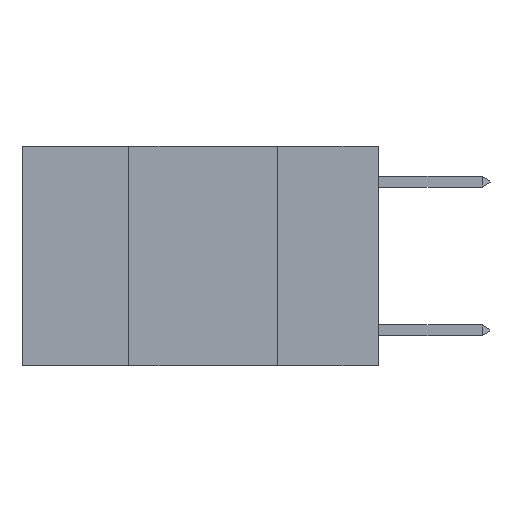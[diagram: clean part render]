
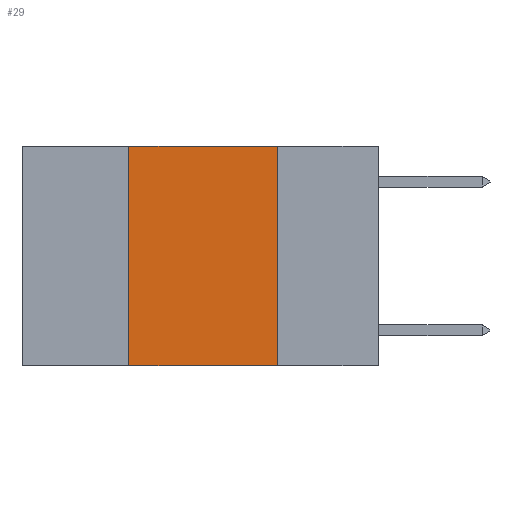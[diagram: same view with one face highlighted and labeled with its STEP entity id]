
A CAD part, left-side view. The second image highlights one B-rep face of the part: STEP entity #29.
In plain terms, the highlighted planar face has unit normal (-1, 0, 0).
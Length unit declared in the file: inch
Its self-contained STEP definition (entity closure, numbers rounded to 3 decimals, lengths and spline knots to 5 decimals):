
#29 = ADVANCED_FACE ( 'NONE', ( #16730 ), #16872, .F. ) ;
#124 = ORIENTED_EDGE ( 'NONE', *, *, #5923, .F. ) ;
#1288 = ORIENTED_EDGE ( 'NONE', *, *, #21244, .T. ) ;
#1526 = VERTEX_POINT ( 'NONE', #14755 ) ;
#2384 = ORIENTED_EDGE ( 'NONE', *, *, #12712, .F. ) ;
#3953 = LINE ( 'NONE', #10150, #18606 ) ;
#3977 = CARTESIAN_POINT ( 'NONE',  ( 0., 0.42, 0. ) ) ;
#5095 = VECTOR ( 'NONE', #12789, 39.37008 ) ;
#5812 = EDGE_LOOP ( 'NONE', ( #2384, #19786, #124, #1288 ) ) ;
#5857 = CARTESIAN_POINT ( 'NONE',  ( 0., 0.17, 0. ) ) ;
#5923 = EDGE_CURVE ( 'NONE', #1526, #10534, #20892, .T. ) ;
#6114 = CARTESIAN_POINT ( 'NONE',  ( 0., 0.17, 0. ) ) ;
#6298 = VERTEX_POINT ( 'NONE', #5857 ) ;
#7700 = EDGE_CURVE ( 'NONE', #10534, #6298, #3953, .T. ) ;
#10044 = DIRECTION ( 'NONE',  ( 0., -1., 0. ) ) ;
#10150 = CARTESIAN_POINT ( 'NONE',  ( 0., 0.6, 0. ) ) ;
#10534 = VERTEX_POINT ( 'NONE', #3977 ) ;
#12712 = EDGE_CURVE ( 'NONE', #6298, #23816, #23791, .T. ) ;
#12789 = DIRECTION ( 'NONE',  ( 0., 0., 1. ) ) ;
#12807 = CARTESIAN_POINT ( 'NONE',  ( 0., 0.42, 0. ) ) ;
#13880 = DIRECTION ( 'NONE',  ( 0., 0., -1. ) ) ;
#14520 = DIRECTION ( 'NONE',  ( 1., 0., 0. ) ) ;
#14755 = CARTESIAN_POINT ( 'NONE',  ( 0., 0.42, -0.37 ) ) ;
#14788 = AXIS2_PLACEMENT_3D ( 'NONE', #15327, #14520, #13880 ) ;
#15327 = CARTESIAN_POINT ( 'NONE',  ( 0., 0.6, 0. ) ) ;
#16730 = FACE_OUTER_BOUND ( 'NONE', #5812, .T. ) ;
#16872 = PLANE ( 'NONE',  #14788 ) ;
#17736 = VECTOR ( 'NONE', #22745, 39.37008 ) ;
#18328 = LINE ( 'NONE', #20777, #17736 ) ;
#18606 = VECTOR ( 'NONE', #10044, 39.37008 ) ;
#18808 = VECTOR ( 'NONE', #21352, 39.37008 ) ;
#19786 = ORIENTED_EDGE ( 'NONE', *, *, #7700, .F. ) ;
#20777 = CARTESIAN_POINT ( 'NONE',  ( 0., 0.6, -0.37 ) ) ;
#20892 = LINE ( 'NONE', #12807, #5095 ) ;
#21244 = EDGE_CURVE ( 'NONE', #1526, #23816, #18328, .T. ) ;
#21352 = DIRECTION ( 'NONE',  ( 0., 0., -1. ) ) ;
#22745 = DIRECTION ( 'NONE',  ( 0., -1., 0. ) ) ;
#23791 = LINE ( 'NONE', #6114, #18808 ) ;
#23816 = VERTEX_POINT ( 'NONE', #24388 ) ;
#24388 = CARTESIAN_POINT ( 'NONE',  ( 0., 0.17, -0.37 ) ) ;
